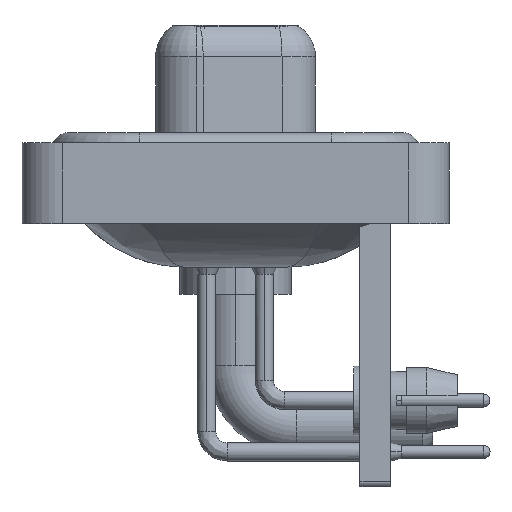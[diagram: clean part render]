
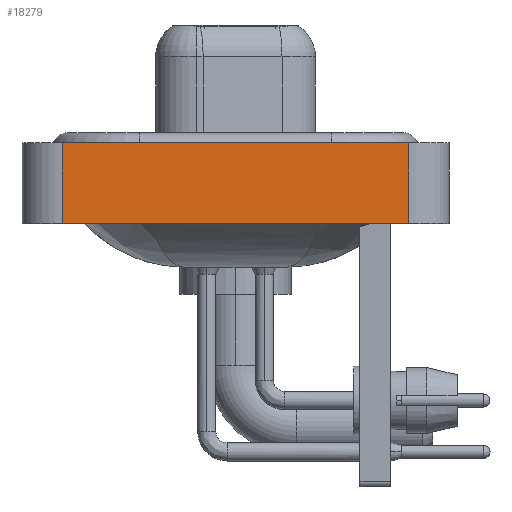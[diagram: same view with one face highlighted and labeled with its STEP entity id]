
A CAD part, left-side view. The second image highlights one B-rep face of the part: STEP entity #18279.
In plain terms, the highlighted planar face has unit normal (-1, 0, 0).
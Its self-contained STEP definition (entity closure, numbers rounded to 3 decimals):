
#375 = LINE ( 'NONE', #5575, #8407 ) ;
#450 = ORIENTED_EDGE ( 'NONE', *, *, #21478, .F. ) ;
#2009 = VERTEX_POINT ( 'NONE', #14845 ) ;
#3516 = DIRECTION ( 'NONE',  ( 0., 0., 1. ) ) ;
#4431 = LINE ( 'NONE', #4545, #8130 ) ;
#4545 = CARTESIAN_POINT ( 'NONE',  ( -7.25, -8.55, -3.6 ) ) ;
#4649 = LINE ( 'NONE', #11423, #9130 ) ;
#4874 = CARTESIAN_POINT ( 'NONE',  ( -7.25, 8.55, -3.6 ) ) ;
#5039 = DIRECTION ( 'NONE',  ( 0., 0., 1. ) ) ;
#5575 = CARTESIAN_POINT ( 'NONE',  ( -7.25, -8.55, 0.4 ) ) ;
#5918 = AXIS2_PLACEMENT_3D ( 'NONE', #18990, #10617, #3516 ) ;
#6601 = CARTESIAN_POINT ( 'NONE',  ( -7.25, -8.55, -3.6 ) ) ;
#6953 = EDGE_CURVE ( 'NONE', #18996, #2009, #4649, .T. ) ;
#7157 = DIRECTION ( 'NONE',  ( 0., -1., 0. ) ) ;
#7540 = VECTOR ( 'NONE', #5039, 1000. ) ;
#7542 = EDGE_LOOP ( 'NONE', ( #14177, #450, #13348, #20438 ) ) ;
#8130 = VECTOR ( 'NONE', #19695, 1000. ) ;
#8407 = VECTOR ( 'NONE', #7157, 1000. ) ;
#8529 = LINE ( 'NONE', #12021, #7540 ) ;
#9130 = VECTOR ( 'NONE', #13127, 1000. ) ;
#10588 = VERTEX_POINT ( 'NONE', #18578 ) ;
#10617 = DIRECTION ( 'NONE',  ( -1., 0., 0. ) ) ;
#11423 = CARTESIAN_POINT ( 'NONE',  ( -7.25, -8.55, -3.6 ) ) ;
#12021 = CARTESIAN_POINT ( 'NONE',  ( -7.25, 8.55, -3.6 ) ) ;
#12090 = PLANE ( 'NONE',  #5918 ) ;
#13127 = DIRECTION ( 'NONE',  ( 0., 0., 1. ) ) ;
#13348 = ORIENTED_EDGE ( 'NONE', *, *, #15861, .F. ) ;
#14177 = ORIENTED_EDGE ( 'NONE', *, *, #6953, .T. ) ;
#14845 = CARTESIAN_POINT ( 'NONE',  ( -7.25, -8.55, 0.4 ) ) ;
#15584 = FACE_OUTER_BOUND ( 'NONE', #7542, .T. ) ;
#15861 = EDGE_CURVE ( 'NONE', #19410, #10588, #8529, .T. ) ;
#18279 = ADVANCED_FACE ( 'NONE', ( #15584 ), #12090, .T. ) ;
#18578 = CARTESIAN_POINT ( 'NONE',  ( -7.25, 8.55, 0.4 ) ) ;
#18990 = CARTESIAN_POINT ( 'NONE',  ( -7.25, -8.55, -3.6 ) ) ;
#18996 = VERTEX_POINT ( 'NONE', #6601 ) ;
#19321 = EDGE_CURVE ( 'NONE', #19410, #18996, #4431, .T. ) ;
#19410 = VERTEX_POINT ( 'NONE', #4874 ) ;
#19695 = DIRECTION ( 'NONE',  ( 0., -1., 0. ) ) ;
#20438 = ORIENTED_EDGE ( 'NONE', *, *, #19321, .T. ) ;
#21478 = EDGE_CURVE ( 'NONE', #10588, #2009, #375, .T. ) ;
